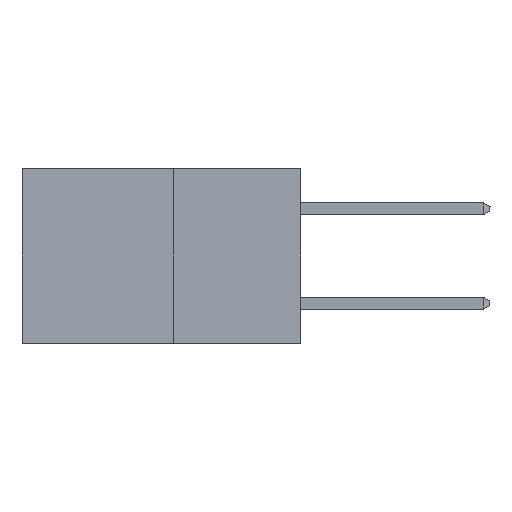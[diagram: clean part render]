
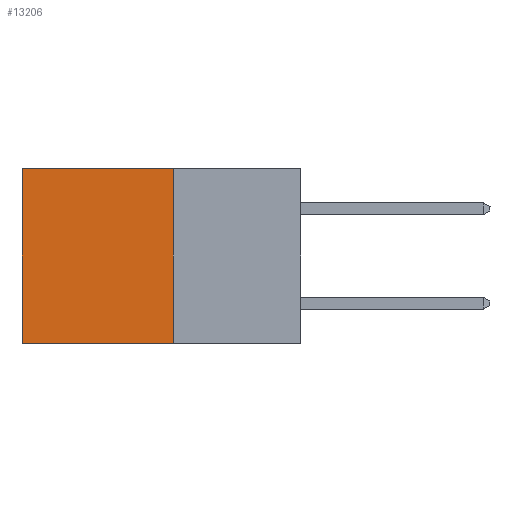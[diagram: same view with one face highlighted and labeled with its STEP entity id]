
A CAD part, left-side view. The second image highlights one B-rep face of the part: STEP entity #13206.
In plain terms, the highlighted planar face has unit normal (-1, 0, 0).
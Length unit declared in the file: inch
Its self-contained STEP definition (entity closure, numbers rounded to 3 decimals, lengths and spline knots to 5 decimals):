
#801 = DIRECTION ( 'NONE',  ( 0., 0., -1. ) ) ;
#1187 = VECTOR ( 'NONE', #15042, 39.37008 ) ;
#1356 = CARTESIAN_POINT ( 'NONE',  ( 0.277, 0.27, -0.37 ) ) ;
#1427 = ORIENTED_EDGE ( 'NONE', *, *, #17303, .T. ) ;
#1441 = EDGE_LOOP ( 'NONE', ( #1427, #9931, #2396, #10866 ) ) ;
#1844 = LINE ( 'NONE', #1356, #10327 ) ;
#2396 = ORIENTED_EDGE ( 'NONE', *, *, #3042, .F. ) ;
#3042 = EDGE_CURVE ( 'NONE', #6200, #6196, #1844, .T. ) ;
#3080 = CARTESIAN_POINT ( 'NONE',  ( 0.277, 0.59, -0.37 ) ) ;
#5165 = CARTESIAN_POINT ( 'NONE',  ( 0.277, 0.27, 0. ) ) ;
#5733 = LINE ( 'NONE', #13831, #13705 ) ;
#6196 = VERTEX_POINT ( 'NONE', #6821 ) ;
#6200 = VERTEX_POINT ( 'NONE', #12765 ) ;
#6373 = DIRECTION ( 'NONE',  ( 0., 1., 0. ) ) ;
#6501 = AXIS2_PLACEMENT_3D ( 'NONE', #8938, #19313, #10443 ) ;
#6683 = DIRECTION ( 'NONE',  ( 0., 1., 0. ) ) ;
#6821 = CARTESIAN_POINT ( 'NONE',  ( 0.277, 0.27, -0.37 ) ) ;
#7374 = EDGE_CURVE ( 'NONE', #6196, #17965, #5733, .T. ) ;
#8067 = CARTESIAN_POINT ( 'NONE',  ( 0.277, 0.59, -0.37 ) ) ;
#8232 = LINE ( 'NONE', #5165, #19146 ) ;
#8938 = CARTESIAN_POINT ( 'NONE',  ( 0.277, 0.27, -0.37 ) ) ;
#9931 = ORIENTED_EDGE ( 'NONE', *, *, #7374, .F. ) ;
#10327 = VECTOR ( 'NONE', #801, 39.37008 ) ;
#10443 = DIRECTION ( 'NONE',  ( 0., 0., -1. ) ) ;
#10866 = ORIENTED_EDGE ( 'NONE', *, *, #18666, .T. ) ;
#12765 = CARTESIAN_POINT ( 'NONE',  ( 0.277, 0.27, 0. ) ) ;
#12812 = FACE_OUTER_BOUND ( 'NONE', #1441, .T. ) ;
#13206 = ADVANCED_FACE ( 'NONE', ( #12812 ), #16375, .F. ) ;
#13705 = VECTOR ( 'NONE', #6373, 39.37008 ) ;
#13831 = CARTESIAN_POINT ( 'NONE',  ( 0.277, 0.27, -0.37 ) ) ;
#14597 = VERTEX_POINT ( 'NONE', #14868 ) ;
#14868 = CARTESIAN_POINT ( 'NONE',  ( 0.277, 0.59, 0. ) ) ;
#15042 = DIRECTION ( 'NONE',  ( 0., 0., -1. ) ) ;
#16375 = PLANE ( 'NONE',  #6501 ) ;
#17151 = LINE ( 'NONE', #3080, #1187 ) ;
#17303 = EDGE_CURVE ( 'NONE', #14597, #17965, #17151, .T. ) ;
#17965 = VERTEX_POINT ( 'NONE', #8067 ) ;
#18666 = EDGE_CURVE ( 'NONE', #6200, #14597, #8232, .T. ) ;
#19146 = VECTOR ( 'NONE', #6683, 39.37008 ) ;
#19313 = DIRECTION ( 'NONE',  ( 1., 0., 0. ) ) ;
